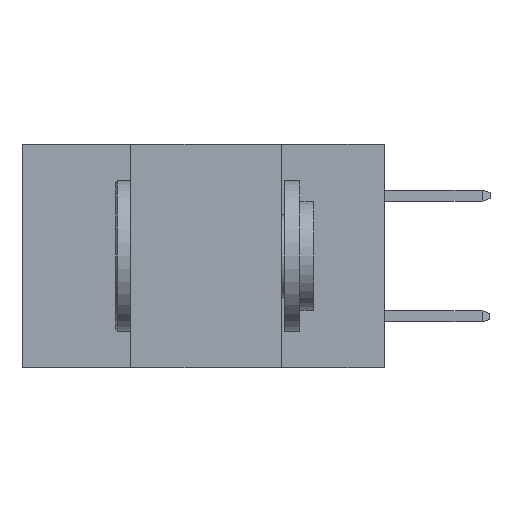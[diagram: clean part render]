
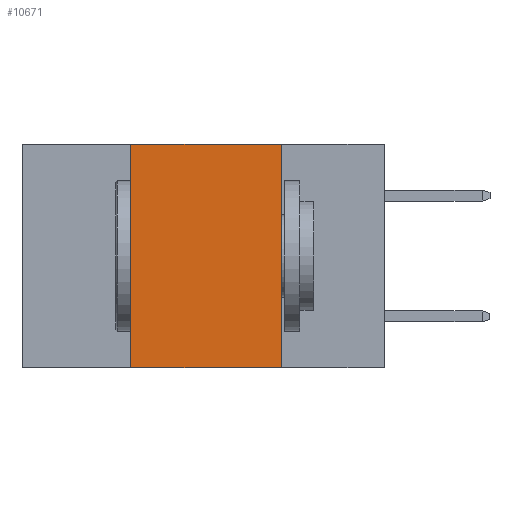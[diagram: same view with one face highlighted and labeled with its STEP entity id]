
A CAD part, left-side view. The second image highlights one B-rep face of the part: STEP entity #10671.
In plain terms, the highlighted planar face has unit normal (-1, 0, 0).
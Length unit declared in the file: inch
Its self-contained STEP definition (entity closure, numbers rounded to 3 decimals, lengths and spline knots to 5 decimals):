
#3 = CARTESIAN_POINT ( 'NONE',  ( 0., 0.42, 0. ) ) ;
#114 = LINE ( 'NONE', #10086, #9005 ) ;
#191 = AXIS2_PLACEMENT_3D ( 'NONE', #5206, #11565, #4726 ) ;
#332 = FACE_OUTER_BOUND ( 'NONE', #5541, .T. ) ;
#561 = ORIENTED_EDGE ( 'NONE', *, *, #1092, .F. ) ;
#763 = LINE ( 'NONE', #2986, #6575 ) ;
#1092 = EDGE_CURVE ( 'NONE', #6658, #10580, #763, .T. ) ;
#1558 = CARTESIAN_POINT ( 'NONE',  ( 0., 0.17, -0.37 ) ) ;
#2013 = DIRECTION ( 'NONE',  ( 0., 0., -1. ) ) ;
#2330 = VECTOR ( 'NONE', #2013, 39.37008 ) ;
#2676 = DIRECTION ( 'NONE',  ( 0., 0., 1. ) ) ;
#2986 = CARTESIAN_POINT ( 'NONE',  ( 0., 0.42, 0. ) ) ;
#3057 = EDGE_CURVE ( 'NONE', #10580, #10969, #11679, .T. ) ;
#3426 = EDGE_CURVE ( 'NONE', #6658, #14448, #114, .T. ) ;
#3567 = PLANE ( 'NONE',  #191 ) ;
#4726 = DIRECTION ( 'NONE',  ( 0., 0., -1. ) ) ;
#5206 = CARTESIAN_POINT ( 'NONE',  ( 0., 0.6, 0. ) ) ;
#5541 = EDGE_LOOP ( 'NONE', ( #11733, #9456, #561, #6751 ) ) ;
#5634 = VECTOR ( 'NONE', #11331, 39.37008 ) ;
#6575 = VECTOR ( 'NONE', #2676, 39.37008 ) ;
#6658 = VERTEX_POINT ( 'NONE', #7993 ) ;
#6751 = ORIENTED_EDGE ( 'NONE', *, *, #3426, .T. ) ;
#7426 = CARTESIAN_POINT ( 'NONE',  ( 0., 0.6, 0. ) ) ;
#7775 = DIRECTION ( 'NONE',  ( 0., -1., 0. ) ) ;
#7993 = CARTESIAN_POINT ( 'NONE',  ( 0., 0.42, -0.37 ) ) ;
#9005 = VECTOR ( 'NONE', #7775, 39.37008 ) ;
#9456 = ORIENTED_EDGE ( 'NONE', *, *, #3057, .F. ) ;
#10038 = CARTESIAN_POINT ( 'NONE',  ( 0., 0.17, 0. ) ) ;
#10086 = CARTESIAN_POINT ( 'NONE',  ( 0., 0.6, -0.37 ) ) ;
#10580 = VERTEX_POINT ( 'NONE', #3 ) ;
#10671 = ADVANCED_FACE ( 'NONE', ( #332 ), #3567, .F. ) ;
#10969 = VERTEX_POINT ( 'NONE', #13103 ) ;
#11110 = EDGE_CURVE ( 'NONE', #10969, #14448, #11453, .T. ) ;
#11331 = DIRECTION ( 'NONE',  ( 0., -1., 0. ) ) ;
#11453 = LINE ( 'NONE', #10038, #2330 ) ;
#11565 = DIRECTION ( 'NONE',  ( 1., 0., 0. ) ) ;
#11679 = LINE ( 'NONE', #7426, #5634 ) ;
#11733 = ORIENTED_EDGE ( 'NONE', *, *, #11110, .F. ) ;
#13103 = CARTESIAN_POINT ( 'NONE',  ( 0., 0.17, 0. ) ) ;
#14448 = VERTEX_POINT ( 'NONE', #1558 ) ;
